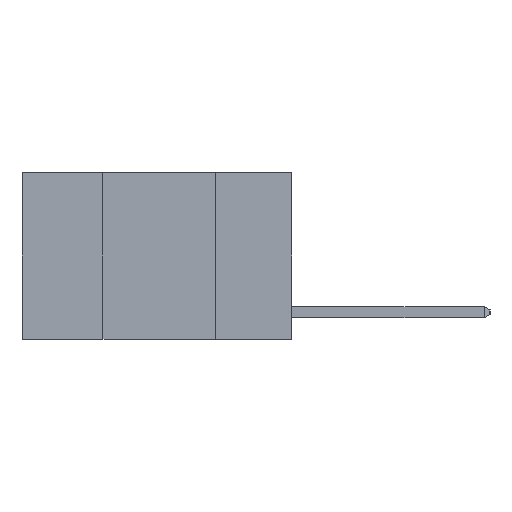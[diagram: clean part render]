
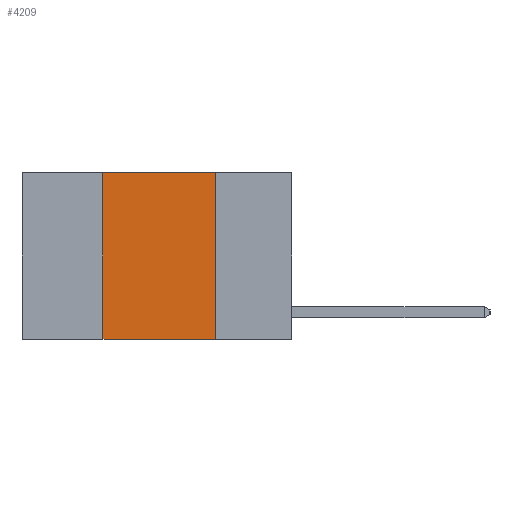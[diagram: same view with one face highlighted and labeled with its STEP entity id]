
A CAD part, left-side view. The second image highlights one B-rep face of the part: STEP entity #4209.
In plain terms, the highlighted planar face has unit normal (-1, 0, 0).
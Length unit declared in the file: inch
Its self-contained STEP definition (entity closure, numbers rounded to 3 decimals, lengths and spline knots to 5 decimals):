
#1084 = PLANE ( 'NONE',  #3276 ) ;
#1173 = VECTOR ( 'NONE', #7149, 39.37008 ) ;
#1360 = VERTEX_POINT ( 'NONE', #4963 ) ;
#1487 = LINE ( 'NONE', #10811, #3710 ) ;
#1488 = EDGE_CURVE ( 'NONE', #4456, #4246, #1487, .T. ) ;
#2062 = DIRECTION ( 'NONE',  ( 0., 0., -1. ) ) ;
#2836 = DIRECTION ( 'NONE',  ( 0., -1., 0. ) ) ;
#3276 = AXIS2_PLACEMENT_3D ( 'NONE', #10478, #7670, #2062 ) ;
#3442 = EDGE_CURVE ( 'NONE', #4456, #6072, #8779, .T. ) ;
#3710 = VECTOR ( 'NONE', #9844, 39.37008 ) ;
#3774 = CARTESIAN_POINT ( 'NONE',  ( 0., 0.6, -0.37 ) ) ;
#3999 = CARTESIAN_POINT ( 'NONE',  ( 0., 0.42, 0. ) ) ;
#4209 = ADVANCED_FACE ( 'NONE', ( #4945 ), #1084, .F. ) ;
#4246 = VERTEX_POINT ( 'NONE', #3999 ) ;
#4331 = CARTESIAN_POINT ( 'NONE',  ( 0., 0.42, -0.37 ) ) ;
#4456 = VERTEX_POINT ( 'NONE', #4331 ) ;
#4525 = ORIENTED_EDGE ( 'NONE', *, *, #7781, .F. ) ;
#4806 = ORIENTED_EDGE ( 'NONE', *, *, #1488, .F. ) ;
#4945 = FACE_OUTER_BOUND ( 'NONE', #7945, .T. ) ;
#4963 = CARTESIAN_POINT ( 'NONE',  ( 0., 0.17, 0. ) ) ;
#6072 = VERTEX_POINT ( 'NONE', #12175 ) ;
#6180 = LINE ( 'NONE', #10926, #1173 ) ;
#6566 = VECTOR ( 'NONE', #2836, 39.37008 ) ;
#6985 = ORIENTED_EDGE ( 'NONE', *, *, #10448, .F. ) ;
#7149 = DIRECTION ( 'NONE',  ( 0., 0., -1. ) ) ;
#7278 = ORIENTED_EDGE ( 'NONE', *, *, #3442, .T. ) ;
#7670 = DIRECTION ( 'NONE',  ( 1., 0., 0. ) ) ;
#7781 = EDGE_CURVE ( 'NONE', #1360, #6072, #6180, .T. ) ;
#7945 = EDGE_LOOP ( 'NONE', ( #4525, #6985, #4806, #7278 ) ) ;
#8779 = LINE ( 'NONE', #3774, #6566 ) ;
#9844 = DIRECTION ( 'NONE',  ( 0., 0., 1. ) ) ;
#10217 = CARTESIAN_POINT ( 'NONE',  ( 0., 0.6, 0. ) ) ;
#10448 = EDGE_CURVE ( 'NONE', #4246, #1360, #11133, .T. ) ;
#10478 = CARTESIAN_POINT ( 'NONE',  ( 0., 0.6, 0. ) ) ;
#10811 = CARTESIAN_POINT ( 'NONE',  ( 0., 0.42, 0. ) ) ;
#10842 = VECTOR ( 'NONE', #12149, 39.37008 ) ;
#10926 = CARTESIAN_POINT ( 'NONE',  ( 0., 0.17, 0. ) ) ;
#11133 = LINE ( 'NONE', #10217, #10842 ) ;
#12149 = DIRECTION ( 'NONE',  ( 0., -1., 0. ) ) ;
#12175 = CARTESIAN_POINT ( 'NONE',  ( 0., 0.17, -0.37 ) ) ;
